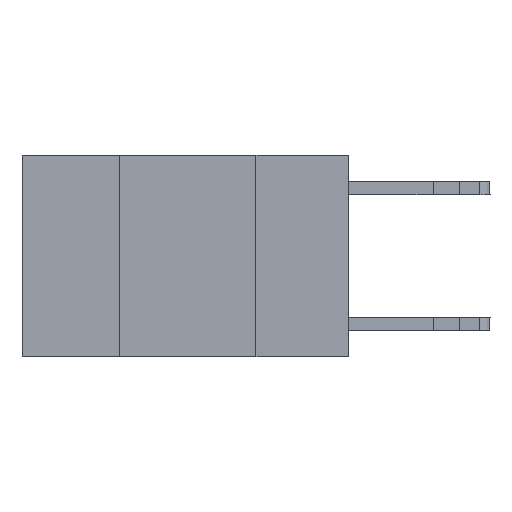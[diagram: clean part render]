
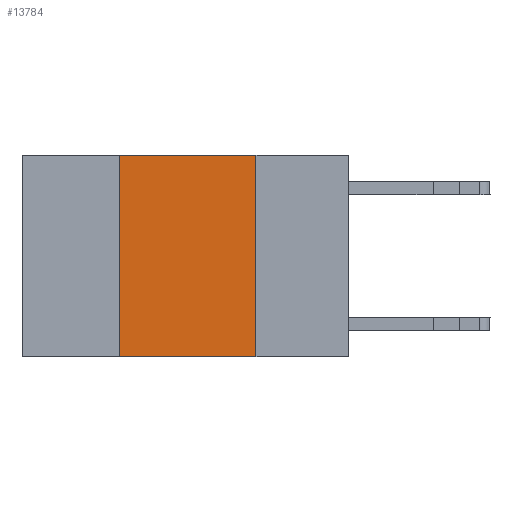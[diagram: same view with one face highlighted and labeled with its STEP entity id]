
A CAD part, left-side view. The second image highlights one B-rep face of the part: STEP entity #13784.
In plain terms, the highlighted planar face has unit normal (-1, 0, 0).
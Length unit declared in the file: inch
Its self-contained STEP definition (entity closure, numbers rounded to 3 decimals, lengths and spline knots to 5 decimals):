
#327 = DIRECTION ( 'NONE',  ( 1., 0., 0. ) ) ;
#1451 = VECTOR ( 'NONE', #15313, 39.37008 ) ;
#1764 = ORIENTED_EDGE ( 'NONE', *, *, #20719, .F. ) ;
#2591 = ORIENTED_EDGE ( 'NONE', *, *, #13113, .F. ) ;
#3182 = EDGE_CURVE ( 'NONE', #11295, #19657, #18016, .T. ) ;
#3288 = CARTESIAN_POINT ( 'NONE',  ( 0., 0.42, 0. ) ) ;
#3394 = EDGE_CURVE ( 'NONE', #11295, #10374, #4259, .T. ) ;
#4016 = VECTOR ( 'NONE', #21017, 39.37008 ) ;
#4259 = LINE ( 'NONE', #18971, #16060 ) ;
#5023 = LINE ( 'NONE', #13498, #20132 ) ;
#5843 = LINE ( 'NONE', #8756, #1451 ) ;
#8066 = DIRECTION ( 'NONE',  ( 0., 0., -1. ) ) ;
#8673 = DIRECTION ( 'NONE',  ( 0., -1., 0. ) ) ;
#8756 = CARTESIAN_POINT ( 'NONE',  ( 0., 0.17, 0. ) ) ;
#8935 = CARTESIAN_POINT ( 'NONE',  ( 0., 0.17, -0.37 ) ) ;
#8940 = ORIENTED_EDGE ( 'NONE', *, *, #3182, .F. ) ;
#10000 = PLANE ( 'NONE',  #17920 ) ;
#10374 = VERTEX_POINT ( 'NONE', #8935 ) ;
#10915 = CARTESIAN_POINT ( 'NONE',  ( 0., 0.42, -0.37 ) ) ;
#11295 = VERTEX_POINT ( 'NONE', #10915 ) ;
#13055 = CARTESIAN_POINT ( 'NONE',  ( 0., 0.17, 0. ) ) ;
#13113 = EDGE_CURVE ( 'NONE', #19228, #10374, #5843, .T. ) ;
#13498 = CARTESIAN_POINT ( 'NONE',  ( 0., 0.6, 0. ) ) ;
#13784 = ADVANCED_FACE ( 'NONE', ( #15063 ), #10000, .F. ) ;
#14823 = ORIENTED_EDGE ( 'NONE', *, *, #3394, .T. ) ;
#14952 = CARTESIAN_POINT ( 'NONE',  ( 0., 0.6, 0. ) ) ;
#15063 = FACE_OUTER_BOUND ( 'NONE', #19550, .T. ) ;
#15313 = DIRECTION ( 'NONE',  ( 0., 0., -1. ) ) ;
#16060 = VECTOR ( 'NONE', #17152, 39.37008 ) ;
#17152 = DIRECTION ( 'NONE',  ( 0., -1., 0. ) ) ;
#17920 = AXIS2_PLACEMENT_3D ( 'NONE', #14952, #327, #8066 ) ;
#18016 = LINE ( 'NONE', #3288, #4016 ) ;
#18971 = CARTESIAN_POINT ( 'NONE',  ( 0., 0.6, -0.37 ) ) ;
#19228 = VERTEX_POINT ( 'NONE', #13055 ) ;
#19550 = EDGE_LOOP ( 'NONE', ( #2591, #1764, #8940, #14823 ) ) ;
#19657 = VERTEX_POINT ( 'NONE', #21149 ) ;
#20132 = VECTOR ( 'NONE', #8673, 39.37008 ) ;
#20719 = EDGE_CURVE ( 'NONE', #19657, #19228, #5023, .T. ) ;
#21017 = DIRECTION ( 'NONE',  ( 0., 0., 1. ) ) ;
#21149 = CARTESIAN_POINT ( 'NONE',  ( 0., 0.42, 0. ) ) ;
